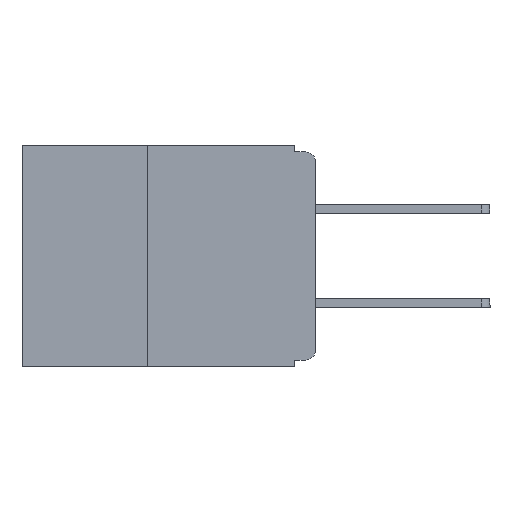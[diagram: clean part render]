
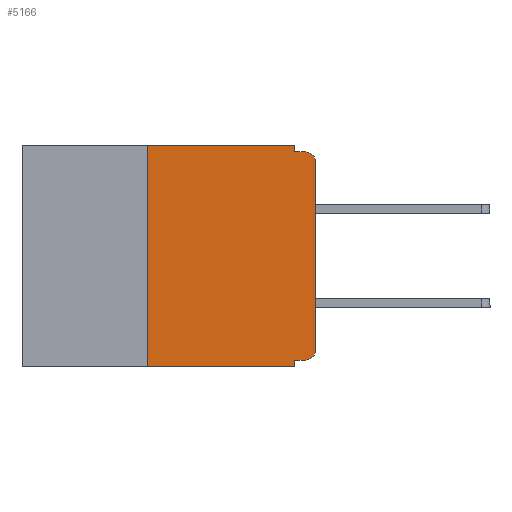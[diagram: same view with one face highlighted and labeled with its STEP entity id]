
A CAD part, left-side view. The second image highlights one B-rep face of the part: STEP entity #5166.
In plain terms, the highlighted planar face has unit normal (-1, 0, 0).
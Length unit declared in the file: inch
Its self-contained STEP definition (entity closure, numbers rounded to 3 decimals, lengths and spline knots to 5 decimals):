
#259 = DIRECTION ( 'NONE',  ( 0., 0., -1. ) ) ;
#454 = CARTESIAN_POINT ( 'NONE',  ( 0., 0.015, -0.025 ) ) ;
#840 = DIRECTION ( 'NONE',  ( 1., 0., 0. ) ) ;
#914 = PLANE ( 'NONE',  #32214 ) ;
#1028 = LINE ( 'NONE', #3516, #21004 ) ;
#1213 = DIRECTION ( 'NONE',  ( 0., 0., -1. ) ) ;
#1443 = VECTOR ( 'NONE', #1213, 39.37008 ) ;
#1635 = CARTESIAN_POINT ( 'NONE',  ( 0., 0.437, 0. ) ) ;
#1640 = ORIENTED_EDGE ( 'NONE', *, *, #14715, .F. ) ;
#1692 = VECTOR ( 'NONE', #20746, 39.37008 ) ;
#3122 = DIRECTION ( 'NONE',  ( 0., 0., -1. ) ) ;
#3350 = LINE ( 'NONE', #15657, #1692 ) ;
#3516 = CARTESIAN_POINT ( 'NONE',  ( 0., 0.437, -0.33 ) ) ;
#3532 = EDGE_CURVE ( 'NONE', #24883, #6380, #20439, .T. ) ;
#3929 = CARTESIAN_POINT ( 'NONE',  ( 0., 0.031, -0.33 ) ) ;
#5166 = ADVANCED_FACE ( 'NONE', ( #31983 ), #914, .F. ) ;
#5732 = VECTOR ( 'NONE', #33239, 39.37008 ) ;
#5969 = EDGE_CURVE ( 'NONE', #26548, #24883, #29954, .T. ) ;
#6380 = VERTEX_POINT ( 'NONE', #33180 ) ;
#6839 = EDGE_CURVE ( 'NONE', #10955, #12691, #8417, .T. ) ;
#7172 = LINE ( 'NONE', #30546, #14092 ) ;
#8417 = LINE ( 'NONE', #9021, #1443 ) ;
#9021 = CARTESIAN_POINT ( 'NONE',  ( 0., 0.031, -0.33 ) ) ;
#9309 = DIRECTION ( 'NONE',  ( 0., 0., -1. ) ) ;
#9444 = EDGE_CURVE ( 'NONE', #6380, #10625, #25282, .T. ) ;
#10176 = LINE ( 'NONE', #27404, #30007 ) ;
#10625 = VERTEX_POINT ( 'NONE', #26316 ) ;
#10663 = LINE ( 'NONE', #14903, #23580 ) ;
#10887 = DIRECTION ( 'NONE',  ( 0., 0., 1. ) ) ;
#10955 = VERTEX_POINT ( 'NONE', #17294 ) ;
#11271 = AXIS2_PLACEMENT_3D ( 'NONE', #12739, #12660, #12622 ) ;
#12065 = CARTESIAN_POINT ( 'NONE',  ( 0., 0., -0.305 ) ) ;
#12201 = AXIS2_PLACEMENT_3D ( 'NONE', #454, #18707, #3122 ) ;
#12398 = ORIENTED_EDGE ( 'NONE', *, *, #13788, .T. ) ;
#12461 = DIRECTION ( 'NONE',  ( 0., 1., 0. ) ) ;
#12515 = ORIENTED_EDGE ( 'NONE', *, *, #6839, .F. ) ;
#12607 = CARTESIAN_POINT ( 'NONE',  ( 0., 0., -0.01 ) ) ;
#12622 = DIRECTION ( 'NONE',  ( 0., 0., -1. ) ) ;
#12633 = LINE ( 'NONE', #12607, #5732 ) ;
#12660 = DIRECTION ( 'NONE',  ( -1., 0., 0. ) ) ;
#12691 = VERTEX_POINT ( 'NONE', #3929 ) ;
#12739 = CARTESIAN_POINT ( 'NONE',  ( 0., 0.015, -0.305 ) ) ;
#13394 = ORIENTED_EDGE ( 'NONE', *, *, #3532, .T. ) ;
#13788 = EDGE_CURVE ( 'NONE', #28802, #12691, #1028, .T. ) ;
#14092 = VECTOR ( 'NONE', #12461, 39.37008 ) ;
#14383 = VECTOR ( 'NONE', #10887, 39.37008 ) ;
#14715 = EDGE_CURVE ( 'NONE', #26548, #10955, #7172, .T. ) ;
#14903 = CARTESIAN_POINT ( 'NONE',  ( 0., 0.25, -0.33 ) ) ;
#15364 = ORIENTED_EDGE ( 'NONE', *, *, #15528, .F. ) ;
#15528 = EDGE_CURVE ( 'NONE', #28802, #32493, #10663, .T. ) ;
#15657 = CARTESIAN_POINT ( 'NONE',  ( 0., 0.437, 0. ) ) ;
#16047 = ORIENTED_EDGE ( 'NONE', *, *, #9444, .T. ) ;
#16386 = CARTESIAN_POINT ( 'NONE',  ( 0., 0., 0. ) ) ;
#17275 = EDGE_CURVE ( 'NONE', #27961, #32462, #10176, .T. ) ;
#17294 = CARTESIAN_POINT ( 'NONE',  ( 0., 0.031, -0.32 ) ) ;
#18707 = DIRECTION ( 'NONE',  ( -1., 0., 0. ) ) ;
#20439 = LINE ( 'NONE', #16386, #14383 ) ;
#20698 = CARTESIAN_POINT ( 'NONE',  ( 0., 0.25, -0.33 ) ) ;
#20746 = DIRECTION ( 'NONE',  ( 0., -1., 0. ) ) ;
#21004 = VECTOR ( 'NONE', #24264, 39.37008 ) ;
#21561 = CARTESIAN_POINT ( 'NONE',  ( 0., 0.031, -0.01 ) ) ;
#22144 = ORIENTED_EDGE ( 'NONE', *, *, #5969, .T. ) ;
#23580 = VECTOR ( 'NONE', #30338, 39.37008 ) ;
#23863 = EDGE_CURVE ( 'NONE', #32493, #27961, #3350, .T. ) ;
#24218 = CARTESIAN_POINT ( 'NONE',  ( 0., 0.25, 0. ) ) ;
#24264 = DIRECTION ( 'NONE',  ( 0., -1., 0. ) ) ;
#24267 = CARTESIAN_POINT ( 'NONE',  ( 0., 0.015, -0.32 ) ) ;
#24458 = ORIENTED_EDGE ( 'NONE', *, *, #23863, .F. ) ;
#24883 = VERTEX_POINT ( 'NONE', #12065 ) ;
#25064 = EDGE_CURVE ( 'NONE', #32462, #10625, #12633, .T. ) ;
#25282 = CIRCLE ( 'NONE', #12201, 0.015 ) ;
#26316 = CARTESIAN_POINT ( 'NONE',  ( 0., 0.015, -0.01 ) ) ;
#26548 = VERTEX_POINT ( 'NONE', #24267 ) ;
#27404 = CARTESIAN_POINT ( 'NONE',  ( 0., 0.031, 0. ) ) ;
#27726 = CARTESIAN_POINT ( 'NONE',  ( 0., 0.031, 0. ) ) ;
#27961 = VERTEX_POINT ( 'NONE', #27726 ) ;
#28338 = EDGE_LOOP ( 'NONE', ( #13394, #16047, #28669, #32146, #24458, #15364, #12398, #12515, #1640, #22144 ) ) ;
#28669 = ORIENTED_EDGE ( 'NONE', *, *, #25064, .F. ) ;
#28802 = VERTEX_POINT ( 'NONE', #20698 ) ;
#29954 = CIRCLE ( 'NONE', #11271, 0.015 ) ;
#30007 = VECTOR ( 'NONE', #9309, 39.37008 ) ;
#30338 = DIRECTION ( 'NONE',  ( 0., 0., 1. ) ) ;
#30546 = CARTESIAN_POINT ( 'NONE',  ( 0., 0., -0.32 ) ) ;
#31983 = FACE_OUTER_BOUND ( 'NONE', #28338, .T. ) ;
#32146 = ORIENTED_EDGE ( 'NONE', *, *, #17275, .F. ) ;
#32214 = AXIS2_PLACEMENT_3D ( 'NONE', #1635, #840, #259 ) ;
#32462 = VERTEX_POINT ( 'NONE', #21561 ) ;
#32493 = VERTEX_POINT ( 'NONE', #24218 ) ;
#33180 = CARTESIAN_POINT ( 'NONE',  ( 0., 0., -0.025 ) ) ;
#33239 = DIRECTION ( 'NONE',  ( 0., -1., 0. ) ) ;
